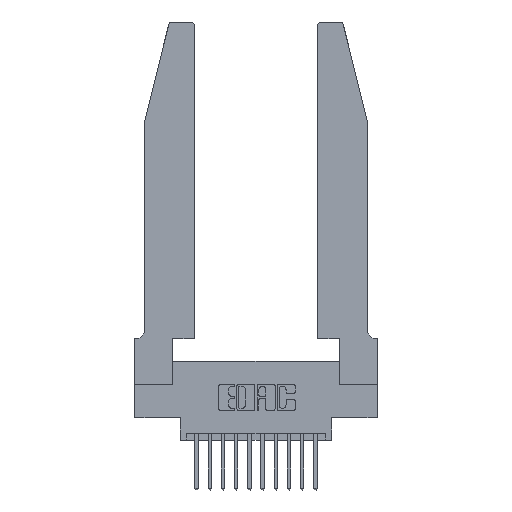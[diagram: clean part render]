
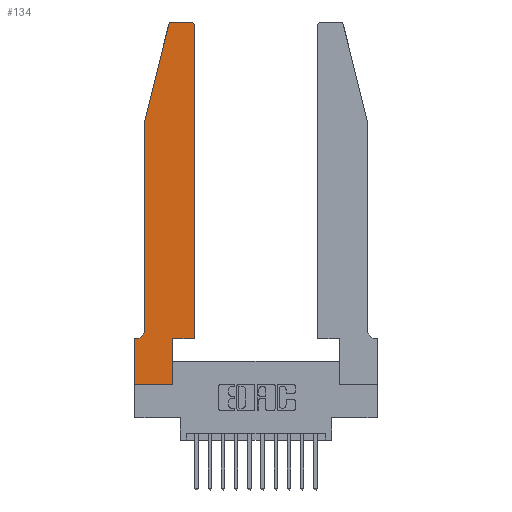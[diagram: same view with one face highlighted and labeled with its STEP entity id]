
A CAD part, top view. The second image highlights one B-rep face of the part: STEP entity #134.
In plain terms, the highlighted planar face has unit normal (0, 0, 1).
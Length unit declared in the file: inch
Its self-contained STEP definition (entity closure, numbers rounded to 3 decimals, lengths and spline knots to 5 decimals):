
#38 = CARTESIAN_POINT ( 'NONE',  ( 0.0755, 2., 0.37 ) ) ;
#134 = ADVANCED_FACE ( 'NONE', ( #16803 ), #988, .T. ) ;
#144 = VECTOR ( 'NONE', #12110, 39.37008 ) ;
#177 = DIRECTION ( 'NONE',  ( 1., 0., 0. ) ) ;
#230 = CARTESIAN_POINT ( 'NONE',  ( 0., 0.35, 0.37 ) ) ;
#249 = DIRECTION ( 'NONE',  ( 0., 0., 1. ) ) ;
#320 = ORIENTED_EDGE ( 'NONE', *, *, #15437, .T. ) ;
#344 = CARTESIAN_POINT ( 'NONE',  ( 0., 0., 0.37 ) ) ;
#697 = DIRECTION ( 'NONE',  ( 0., 1., 0. ) ) ;
#746 = ORIENTED_EDGE ( 'NONE', *, *, #16552, .T. ) ;
#871 = VERTEX_POINT ( 'NONE', #5168 ) ;
#976 = DIRECTION ( 'NONE',  ( 0., -1., 0. ) ) ;
#988 = PLANE ( 'NONE',  #1920 ) ;
#1239 = CARTESIAN_POINT ( 'NONE',  ( 0.0055, 0.42, 0.37 ) ) ;
#1426 = EDGE_CURVE ( 'NONE', #15542, #10125, #12252, .T. ) ;
#1447 = DIRECTION ( 'NONE',  ( 0., -1., 0. ) ) ;
#1525 = DIRECTION ( 'NONE',  ( 1., 0., 0. ) ) ;
#1598 = DIRECTION ( 'NONE',  ( 0., 0., 1. ) ) ;
#1639 = AXIS2_PLACEMENT_3D ( 'NONE', #1239, #10663, #2629 ) ;
#1820 = ORIENTED_EDGE ( 'NONE', *, *, #9095, .T. ) ;
#1920 = AXIS2_PLACEMENT_3D ( 'NONE', #230, #249, #1525 ) ;
#2147 = VECTOR ( 'NONE', #177, 39.37008 ) ;
#2463 = CIRCLE ( 'NONE', #11054, 0.03 ) ;
#2466 = VECTOR ( 'NONE', #10897, 39.37008 ) ;
#2629 = DIRECTION ( 'NONE',  ( -1., 0., 0. ) ) ;
#3116 = EDGE_LOOP ( 'NONE', ( #12066, #1820, #9017, #5896, #9456, #6305, #9871, #10265, #10674, #14039, #320, #746 ) ) ;
#3246 = CARTESIAN_POINT ( 'NONE',  ( 0.4205, 2.72, 0.37 ) ) ;
#3359 = VECTOR ( 'NONE', #8486, 39.37008 ) ;
#3707 = CARTESIAN_POINT ( 'NONE',  ( 0., 0., 0.37 ) ) ;
#3841 = VECTOR ( 'NONE', #15772, 39.37008 ) ;
#3909 = CARTESIAN_POINT ( 'NONE',  ( 0.4505, 0.35, 0.37 ) ) ;
#4243 = EDGE_CURVE ( 'NONE', #9518, #14756, #5798, .T. ) ;
#4276 = LINE ( 'NONE', #14512, #3841 ) ;
#4346 = VECTOR ( 'NONE', #11185, 39.37008 ) ;
#4620 = DIRECTION ( 'NONE',  ( 1., 0., 0. ) ) ;
#4803 = EDGE_CURVE ( 'NONE', #13244, #8974, #15285, .T. ) ;
#4871 = VERTEX_POINT ( 'NONE', #5694 ) ;
#4979 = EDGE_CURVE ( 'NONE', #13280, #9665, #7914, .T. ) ;
#5004 = CARTESIAN_POINT ( 'NONE',  ( 0.2865, 0., 0.37 ) ) ;
#5008 = CARTESIAN_POINT ( 'NONE',  ( 0.2865, 0.35, 0.37 ) ) ;
#5168 = CARTESIAN_POINT ( 'NONE',  ( 0.4505, 2.72, 0.37 ) ) ;
#5230 = VECTOR ( 'NONE', #976, 39.37008 ) ;
#5694 = CARTESIAN_POINT ( 'NONE',  ( 0.25487, 2.72718, 0.37 ) ) ;
#5798 = LINE ( 'NONE', #8345, #2147 ) ;
#5896 = ORIENTED_EDGE ( 'NONE', *, *, #4803, .T. ) ;
#6305 = ORIENTED_EDGE ( 'NONE', *, *, #1426, .T. ) ;
#6693 = AXIS2_PLACEMENT_3D ( 'NONE', #3246, #12495, #4620 ) ;
#7144 = LINE ( 'NONE', #16467, #13651 ) ;
#7294 = CIRCLE ( 'NONE', #1639, 0.07 ) ;
#7408 = LINE ( 'NONE', #9533, #144 ) ;
#7520 = EDGE_CURVE ( 'NONE', #4871, #13244, #7408, .T. ) ;
#7594 = CARTESIAN_POINT ( 'NONE',  ( 0.4205, 2.75, 0.37 ) ) ;
#7914 = LINE ( 'NONE', #9900, #4346 ) ;
#8345 = CARTESIAN_POINT ( 'NONE',  ( 0.4505, 0.35, 0.37 ) ) ;
#8486 = DIRECTION ( 'NONE',  ( 1., 0., 0. ) ) ;
#8534 = EDGE_CURVE ( 'NONE', #9948, #13335, #13051, .T. ) ;
#8737 = EDGE_CURVE ( 'NONE', #13335, #9518, #7144, .T. ) ;
#8752 = CARTESIAN_POINT ( 'NONE',  ( 0.0755, 2., 0.37 ) ) ;
#8974 = VERTEX_POINT ( 'NONE', #15726 ) ;
#9017 = ORIENTED_EDGE ( 'NONE', *, *, #7520, .T. ) ;
#9095 = EDGE_CURVE ( 'NONE', #9665, #4871, #2463, .T. ) ;
#9456 = ORIENTED_EDGE ( 'NONE', *, *, #12868, .T. ) ;
#9518 = VERTEX_POINT ( 'NONE', #5008 ) ;
#9533 = CARTESIAN_POINT ( 'NONE',  ( 0.0755, 2., 0.37 ) ) ;
#9548 = EDGE_CURVE ( 'NONE', #10125, #9948, #15570, .T. ) ;
#9665 = VERTEX_POINT ( 'NONE', #10588 ) ;
#9712 = CARTESIAN_POINT ( 'NONE',  ( 0.284, 2.72, 0.37 ) ) ;
#9871 = ORIENTED_EDGE ( 'NONE', *, *, #9548, .T. ) ;
#9900 = CARTESIAN_POINT ( 'NONE',  ( 0.2605, 2.75, 0.37 ) ) ;
#9948 = VERTEX_POINT ( 'NONE', #12405 ) ;
#10125 = VERTEX_POINT ( 'NONE', #13004 ) ;
#10265 = ORIENTED_EDGE ( 'NONE', *, *, #8534, .T. ) ;
#10588 = CARTESIAN_POINT ( 'NONE',  ( 0.284, 2.75, 0.37 ) ) ;
#10663 = DIRECTION ( 'NONE',  ( 0., 0., -1. ) ) ;
#10674 = ORIENTED_EDGE ( 'NONE', *, *, #8737, .T. ) ;
#10897 = DIRECTION ( 'NONE',  ( -1., 0., 0. ) ) ;
#10997 = DIRECTION ( 'NONE',  ( 1., 0., 0. ) ) ;
#11054 = AXIS2_PLACEMENT_3D ( 'NONE', #9712, #1598, #10997 ) ;
#11185 = DIRECTION ( 'NONE',  ( -1., 0., 0. ) ) ;
#12066 = ORIENTED_EDGE ( 'NONE', *, *, #4979, .T. ) ;
#12110 = DIRECTION ( 'NONE',  ( -0.239, -0.971, 0. ) ) ;
#12252 = LINE ( 'NONE', #15367, #2466 ) ;
#12276 = CIRCLE ( 'NONE', #6693, 0.03 ) ;
#12405 = CARTESIAN_POINT ( 'NONE',  ( 0., 0., 0.37 ) ) ;
#12495 = DIRECTION ( 'NONE',  ( 0., 0., 1. ) ) ;
#12868 = EDGE_CURVE ( 'NONE', #8974, #15542, #7294, .T. ) ;
#13004 = CARTESIAN_POINT ( 'NONE',  ( 0., 0.35, 0.37 ) ) ;
#13051 = LINE ( 'NONE', #344, #3359 ) ;
#13244 = VERTEX_POINT ( 'NONE', #8752 ) ;
#13280 = VERTEX_POINT ( 'NONE', #7594 ) ;
#13335 = VERTEX_POINT ( 'NONE', #5004 ) ;
#13422 = CARTESIAN_POINT ( 'NONE',  ( 0.0055, 0.35, 0.37 ) ) ;
#13651 = VECTOR ( 'NONE', #697, 39.37008 ) ;
#14039 = ORIENTED_EDGE ( 'NONE', *, *, #4243, .T. ) ;
#14512 = CARTESIAN_POINT ( 'NONE',  ( 0.4505, 0.35, 0.37 ) ) ;
#14756 = VERTEX_POINT ( 'NONE', #3909 ) ;
#14889 = VECTOR ( 'NONE', #1447, 39.37008 ) ;
#15285 = LINE ( 'NONE', #38, #14889 ) ;
#15367 = CARTESIAN_POINT ( 'NONE',  ( 0.0755, 0.35, 0.37 ) ) ;
#15437 = EDGE_CURVE ( 'NONE', #14756, #871, #4276, .T. ) ;
#15542 = VERTEX_POINT ( 'NONE', #13422 ) ;
#15570 = LINE ( 'NONE', #3707, #5230 ) ;
#15726 = CARTESIAN_POINT ( 'NONE',  ( 0.0755, 0.42, 0.37 ) ) ;
#15772 = DIRECTION ( 'NONE',  ( 0., 1., 0. ) ) ;
#16467 = CARTESIAN_POINT ( 'NONE',  ( 0.2865, 0.35, 0.37 ) ) ;
#16552 = EDGE_CURVE ( 'NONE', #871, #13280, #12276, .T. ) ;
#16803 = FACE_OUTER_BOUND ( 'NONE', #3116, .T. ) ;
